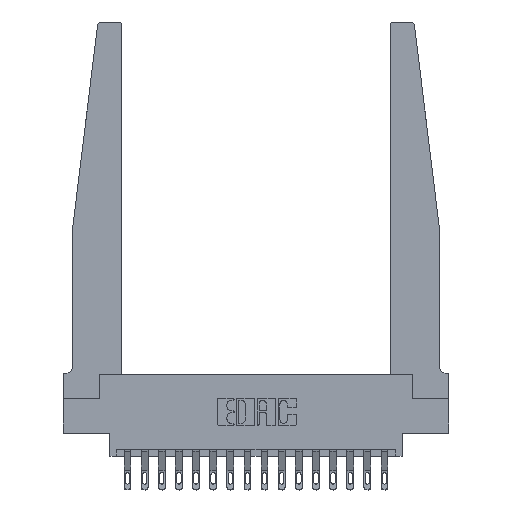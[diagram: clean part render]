
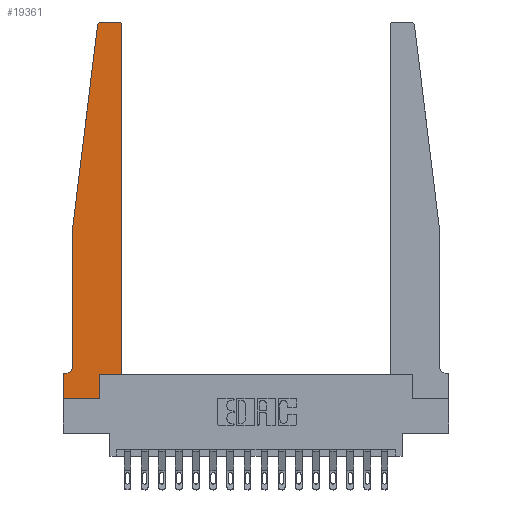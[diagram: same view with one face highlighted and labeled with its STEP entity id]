
A CAD part, top view. The second image highlights one B-rep face of the part: STEP entity #19361.
In plain terms, the highlighted planar face has unit normal (0, 0, 1).
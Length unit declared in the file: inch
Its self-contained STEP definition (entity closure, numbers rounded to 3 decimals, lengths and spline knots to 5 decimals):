
#18 = DIRECTION ( 'NONE',  ( -1., 0., 0. ) ) ;
#199 = EDGE_CURVE ( 'NONE', #16282, #9582, #10844, .T. ) ;
#602 = VECTOR ( 'NONE', #6318, 39.37008 ) ;
#946 = VERTEX_POINT ( 'NONE', #7805 ) ;
#1151 = EDGE_CURVE ( 'NONE', #3020, #13463, #5715, .T. ) ;
#1176 = DIRECTION ( 'NONE',  ( 0., 0., 1. ) ) ;
#1562 = ORIENTED_EDGE ( 'NONE', *, *, #6570, .T. ) ;
#1695 = EDGE_CURVE ( 'NONE', #9582, #3097, #6268, .T. ) ;
#2006 = CARTESIAN_POINT ( 'NONE',  ( 0.065, 0.2375, 0.37 ) ) ;
#2386 = DIRECTION ( 'NONE',  ( 1., 0., 0. ) ) ;
#2750 = CARTESIAN_POINT ( 'NONE',  ( 0.27653, 2.75, 0.37 ) ) ;
#2781 = AXIS2_PLACEMENT_3D ( 'NONE', #17504, #8621, #19295 ) ;
#2811 = VECTOR ( 'NONE', #18207, 39.37008 ) ;
#2872 = DIRECTION ( 'NONE',  ( 1., 0., 0. ) ) ;
#3020 = VERTEX_POINT ( 'NONE', #10905 ) ;
#3097 = VERTEX_POINT ( 'NONE', #18823 ) ;
#3366 = EDGE_CURVE ( 'NONE', #3097, #9554, #15299, .T. ) ;
#3476 = EDGE_CURVE ( 'NONE', #13463, #5060, #18679, .T. ) ;
#3722 = ORIENTED_EDGE ( 'NONE', *, *, #15577, .T. ) ;
#4636 = CIRCLE ( 'NONE', #2781, 0.03 ) ;
#4792 = VERTEX_POINT ( 'NONE', #5024 ) ;
#4945 = VERTEX_POINT ( 'NONE', #16671 ) ;
#4972 = EDGE_CURVE ( 'NONE', #4945, #16282, #16769, .T. ) ;
#5024 = CARTESIAN_POINT ( 'NONE',  ( 0.425, 2.72, 0.37 ) ) ;
#5060 = VERTEX_POINT ( 'NONE', #11523 ) ;
#5074 = EDGE_CURVE ( 'NONE', #5060, #4792, #17541, .T. ) ;
#5557 = CARTESIAN_POINT ( 'NONE',  ( 0., 0.1875, 0.37 ) ) ;
#5715 = LINE ( 'NONE', #17874, #13599 ) ;
#5939 = VECTOR ( 'NONE', #12438, 39.37008 ) ;
#5974 = ORIENTED_EDGE ( 'NONE', *, *, #5074, .T. ) ;
#6268 = LINE ( 'NONE', #9166, #11122 ) ;
#6290 = DIRECTION ( 'NONE',  ( 0., -1., 0. ) ) ;
#6318 = DIRECTION ( 'NONE',  ( -1., 0., 0. ) ) ;
#6420 = LINE ( 'NONE', #12452, #602 ) ;
#6524 = ORIENTED_EDGE ( 'NONE', *, *, #8971, .T. ) ;
#6570 = EDGE_CURVE ( 'NONE', #10680, #3020, #13409, .T. ) ;
#7221 = VERTEX_POINT ( 'NONE', #5557 ) ;
#7805 = CARTESIAN_POINT ( 'NONE',  ( 0.015, 0.1875, 0.37 ) ) ;
#7839 = EDGE_LOOP ( 'NONE', ( #11482, #14059, #10849, #18350, #13662, #3722, #6524, #1562, #13786, #15147, #5974, #15593 ) ) ;
#8251 = VECTOR ( 'NONE', #6290, 39.37008 ) ;
#8254 = CARTESIAN_POINT ( 'NONE',  ( 0.015, 0.2375, 0.37 ) ) ;
#8621 = DIRECTION ( 'NONE',  ( 0., 0., 1. ) ) ;
#8802 = VECTOR ( 'NONE', #18, 39.37008 ) ;
#8971 = EDGE_CURVE ( 'NONE', #7221, #10680, #9415, .T. ) ;
#9166 = CARTESIAN_POINT ( 'NONE',  ( 0.065, 1.25, 0.37 ) ) ;
#9415 = LINE ( 'NONE', #12181, #2811 ) ;
#9554 = VERTEX_POINT ( 'NONE', #2006 ) ;
#9582 = VERTEX_POINT ( 'NONE', #18687 ) ;
#9931 = CARTESIAN_POINT ( 'NONE',  ( 0.2605, 0.18, 0.37 ) ) ;
#10680 = VERTEX_POINT ( 'NONE', #15788 ) ;
#10844 = CIRCLE ( 'NONE', #15887, 0.03 ) ;
#10849 = ORIENTED_EDGE ( 'NONE', *, *, #1695, .T. ) ;
#10856 = CARTESIAN_POINT ( 'NONE',  ( 0.065, 1.25, 0.37 ) ) ;
#10905 = CARTESIAN_POINT ( 'NONE',  ( 0.2605, 0., 0.37 ) ) ;
#10954 = CARTESIAN_POINT ( 'NONE',  ( 0.425, 0.18, 0.37 ) ) ;
#11122 = VECTOR ( 'NONE', #13502, 39.37008 ) ;
#11482 = ORIENTED_EDGE ( 'NONE', *, *, #4972, .T. ) ;
#11523 = CARTESIAN_POINT ( 'NONE',  ( 0.425, 0.18, 0.37 ) ) ;
#11617 = CARTESIAN_POINT ( 'NONE',  ( 0., 0.1875, 0.37 ) ) ;
#11999 = CIRCLE ( 'NONE', #18646, 0.05 ) ;
#12181 = CARTESIAN_POINT ( 'NONE',  ( 0., 0., 0.37 ) ) ;
#12268 = EDGE_CURVE ( 'NONE', #4792, #4945, #4636, .T. ) ;
#12329 = DIRECTION ( 'NONE',  ( 0., 0., 1. ) ) ;
#12351 = VECTOR ( 'NONE', #2386, 39.37008 ) ;
#12438 = DIRECTION ( 'NONE',  ( 0., 1., 0. ) ) ;
#12452 = CARTESIAN_POINT ( 'NONE',  ( 0.065, 0.1875, 0.37 ) ) ;
#13409 = LINE ( 'NONE', #19546, #18761 ) ;
#13431 = CARTESIAN_POINT ( 'NONE',  ( 0.25, 2.75, 0.37 ) ) ;
#13463 = VERTEX_POINT ( 'NONE', #9931 ) ;
#13502 = DIRECTION ( 'NONE',  ( -0.122, -0.992, 0. ) ) ;
#13599 = VECTOR ( 'NONE', #19380, 39.37008 ) ;
#13662 = ORIENTED_EDGE ( 'NONE', *, *, #14880, .T. ) ;
#13786 = ORIENTED_EDGE ( 'NONE', *, *, #1151, .T. ) ;
#14059 = ORIENTED_EDGE ( 'NONE', *, *, #199, .T. ) ;
#14382 = DIRECTION ( 'NONE',  ( -1., 0., 0. ) ) ;
#14880 = EDGE_CURVE ( 'NONE', #9554, #946, #11999, .T. ) ;
#15147 = ORIENTED_EDGE ( 'NONE', *, *, #3476, .T. ) ;
#15299 = LINE ( 'NONE', #10856, #8251 ) ;
#15577 = EDGE_CURVE ( 'NONE', #946, #7221, #6420, .T. ) ;
#15593 = ORIENTED_EDGE ( 'NONE', *, *, #12268, .T. ) ;
#15788 = CARTESIAN_POINT ( 'NONE',  ( 0., 0., 0.37 ) ) ;
#15875 = CARTESIAN_POINT ( 'NONE',  ( 0.425, 0.18, 0.37 ) ) ;
#15887 = AXIS2_PLACEMENT_3D ( 'NONE', #18169, #12329, #19557 ) ;
#16038 = DIRECTION ( 'NONE',  ( 0., 0., -1. ) ) ;
#16052 = PLANE ( 'NONE',  #17117 ) ;
#16282 = VERTEX_POINT ( 'NONE', #2750 ) ;
#16671 = CARTESIAN_POINT ( 'NONE',  ( 0.395, 2.75, 0.37 ) ) ;
#16769 = LINE ( 'NONE', #13431, #8802 ) ;
#17117 = AXIS2_PLACEMENT_3D ( 'NONE', #11617, #1176, #2872 ) ;
#17504 = CARTESIAN_POINT ( 'NONE',  ( 0.395, 2.72, 0.37 ) ) ;
#17541 = LINE ( 'NONE', #10954, #5939 ) ;
#17861 = DIRECTION ( 'NONE',  ( 1., 0., 0. ) ) ;
#17874 = CARTESIAN_POINT ( 'NONE',  ( 0.2605, 0.18, 0.37 ) ) ;
#17934 = FACE_OUTER_BOUND ( 'NONE', #7839, .T. ) ;
#18169 = CARTESIAN_POINT ( 'NONE',  ( 0.27653, 2.72, 0.37 ) ) ;
#18207 = DIRECTION ( 'NONE',  ( 0., -1., 0. ) ) ;
#18350 = ORIENTED_EDGE ( 'NONE', *, *, #3366, .T. ) ;
#18646 = AXIS2_PLACEMENT_3D ( 'NONE', #8254, #16038, #14382 ) ;
#18679 = LINE ( 'NONE', #15875, #12351 ) ;
#18687 = CARTESIAN_POINT ( 'NONE',  ( 0.24675, 2.72367, 0.37 ) ) ;
#18761 = VECTOR ( 'NONE', #17861, 39.37008 ) ;
#18823 = CARTESIAN_POINT ( 'NONE',  ( 0.065, 1.25, 0.37 ) ) ;
#19295 = DIRECTION ( 'NONE',  ( 1., 0., 0. ) ) ;
#19361 = ADVANCED_FACE ( 'NONE', ( #17934 ), #16052, .T. ) ;
#19380 = DIRECTION ( 'NONE',  ( 0., 1., 0. ) ) ;
#19546 = CARTESIAN_POINT ( 'NONE',  ( 0., 0., 0.37 ) ) ;
#19557 = DIRECTION ( 'NONE',  ( 1., 0., 0. ) ) ;
